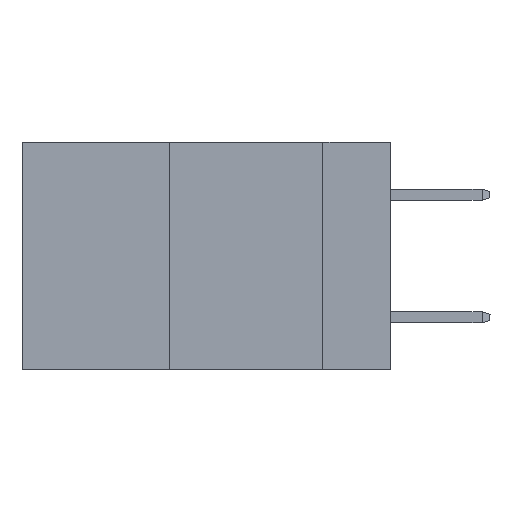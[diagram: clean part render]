
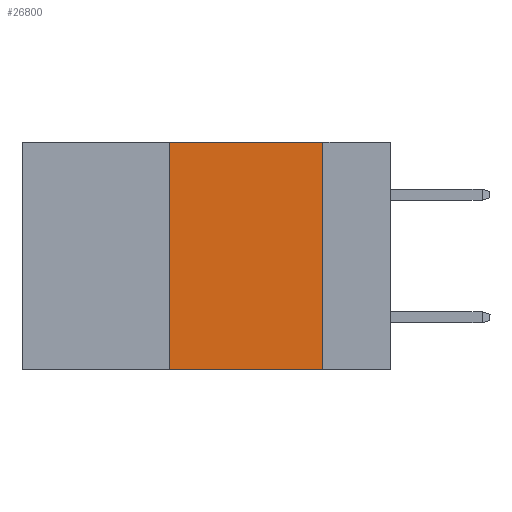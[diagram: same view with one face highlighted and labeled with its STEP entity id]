
A CAD part, left-side view. The second image highlights one B-rep face of the part: STEP entity #26800.
In plain terms, the highlighted planar face has unit normal (-1, 0, 0).
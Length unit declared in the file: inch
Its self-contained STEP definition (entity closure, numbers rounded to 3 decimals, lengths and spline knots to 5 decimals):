
#1651 = CARTESIAN_POINT ( 'NONE',  ( 0., 0.11, 0. ) ) ;
#4896 = CARTESIAN_POINT ( 'NONE',  ( 0., 0.11, 0. ) ) ;
#10266 = VERTEX_POINT ( 'NONE', #38394 ) ;
#11092 = VECTOR ( 'NONE', #41142, 39.37008 ) ;
#11316 = EDGE_LOOP ( 'NONE', ( #28557, #32021, #29318, #18959 ) ) ;
#13443 = CARTESIAN_POINT ( 'NONE',  ( 0., 0.6, 0. ) ) ;
#14028 = LINE ( 'NONE', #21787, #27494 ) ;
#14876 = VECTOR ( 'NONE', #34758, 39.37008 ) ;
#16344 = PLANE ( 'NONE',  #23656 ) ;
#16975 = DIRECTION ( 'NONE',  ( 0., -1., 0. ) ) ;
#18959 = ORIENTED_EDGE ( 'NONE', *, *, #28802, .T. ) ;
#19188 = EDGE_CURVE ( 'NONE', #28122, #10266, #42743, .T. ) ;
#20089 = LINE ( 'NONE', #31018, #14876 ) ;
#21787 = CARTESIAN_POINT ( 'NONE',  ( 0., 0.36, 0. ) ) ;
#22905 = DIRECTION ( 'NONE',  ( 0., 0., -1. ) ) ;
#23656 = AXIS2_PLACEMENT_3D ( 'NONE', #13443, #36625, #22905 ) ;
#23707 = VECTOR ( 'NONE', #16975, 39.37008 ) ;
#24431 = EDGE_CURVE ( 'NONE', #35828, #28122, #30403, .T. ) ;
#26585 = EDGE_CURVE ( 'NONE', #26832, #35828, #14028, .T. ) ;
#26800 = ADVANCED_FACE ( 'NONE', ( #30054 ), #16344, .F. ) ;
#26832 = VERTEX_POINT ( 'NONE', #36766 ) ;
#27494 = VECTOR ( 'NONE', #32579, 39.37008 ) ;
#28122 = VERTEX_POINT ( 'NONE', #1651 ) ;
#28557 = ORIENTED_EDGE ( 'NONE', *, *, #19188, .F. ) ;
#28802 = EDGE_CURVE ( 'NONE', #26832, #10266, #20089, .T. ) ;
#29318 = ORIENTED_EDGE ( 'NONE', *, *, #26585, .F. ) ;
#30054 = FACE_OUTER_BOUND ( 'NONE', #11316, .T. ) ;
#30403 = LINE ( 'NONE', #40166, #23707 ) ;
#31018 = CARTESIAN_POINT ( 'NONE',  ( 0., 0.6, -0.37 ) ) ;
#32021 = ORIENTED_EDGE ( 'NONE', *, *, #24431, .F. ) ;
#32579 = DIRECTION ( 'NONE',  ( 0., 0., 1. ) ) ;
#34758 = DIRECTION ( 'NONE',  ( 0., -1., 0. ) ) ;
#35828 = VERTEX_POINT ( 'NONE', #42677 ) ;
#36625 = DIRECTION ( 'NONE',  ( 1., 0., 0. ) ) ;
#36766 = CARTESIAN_POINT ( 'NONE',  ( 0., 0.36, -0.37 ) ) ;
#38394 = CARTESIAN_POINT ( 'NONE',  ( 0., 0.11, -0.37 ) ) ;
#40166 = CARTESIAN_POINT ( 'NONE',  ( 0., 0.6, 0. ) ) ;
#41142 = DIRECTION ( 'NONE',  ( 0., 0., -1. ) ) ;
#42677 = CARTESIAN_POINT ( 'NONE',  ( 0., 0.36, 0. ) ) ;
#42743 = LINE ( 'NONE', #4896, #11092 ) ;
